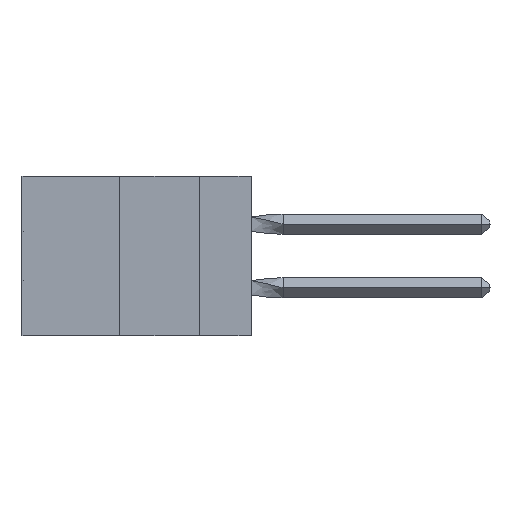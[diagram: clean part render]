
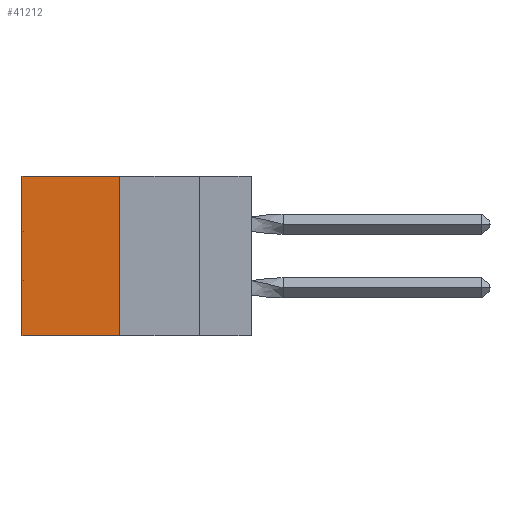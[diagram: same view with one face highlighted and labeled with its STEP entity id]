
A CAD part, left-side view. The second image highlights one B-rep face of the part: STEP entity #41212.
In plain terms, the highlighted planar face has unit normal (-1, 0, 0).
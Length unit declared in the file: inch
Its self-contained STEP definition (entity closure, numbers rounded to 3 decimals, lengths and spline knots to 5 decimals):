
#1384 = VERTEX_POINT ( 'NONE', #13139 ) ;
#1548 = LINE ( 'NONE', #21784, #15358 ) ;
#1562 = EDGE_CURVE ( 'NONE', #7573, #21816, #4903, .T. ) ;
#2944 = DIRECTION ( 'NONE',  ( 0., 0., -1. ) ) ;
#3630 = LINE ( 'NONE', #15816, #15417 ) ;
#4903 = LINE ( 'NONE', #5093, #20805 ) ;
#4969 = EDGE_LOOP ( 'NONE', ( #41977, #9953, #30046, #12550 ) ) ;
#5093 = CARTESIAN_POINT ( 'NONE',  ( 0.305, 0.413, -0.5 ) ) ;
#7357 = DIRECTION ( 'NONE',  ( 0., 0., -1. ) ) ;
#7573 = VERTEX_POINT ( 'NONE', #14237 ) ;
#8630 = DIRECTION ( 'NONE',  ( 0., 0., -1. ) ) ;
#9953 = ORIENTED_EDGE ( 'NONE', *, *, #1562, .F. ) ;
#12550 = ORIENTED_EDGE ( 'NONE', *, *, #19380, .T. ) ;
#12794 = DIRECTION ( 'NONE',  ( 1., 0., 0. ) ) ;
#13139 = CARTESIAN_POINT ( 'NONE',  ( 0.305, 0.72, 0. ) ) ;
#14204 = CARTESIAN_POINT ( 'NONE',  ( 0.305, 0.72, -0.5 ) ) ;
#14237 = CARTESIAN_POINT ( 'NONE',  ( 0.305, 0.413, -0.5 ) ) ;
#14244 = AXIS2_PLACEMENT_3D ( 'NONE', #20266, #12794, #7357 ) ;
#15358 = VECTOR ( 'NONE', #8630, 39.37008 ) ;
#15417 = VECTOR ( 'NONE', #2944, 39.37008 ) ;
#15816 = CARTESIAN_POINT ( 'NONE',  ( 0.305, 0.72, -0.5 ) ) ;
#19380 = EDGE_CURVE ( 'NONE', #39048, #1384, #26213, .T. ) ;
#20266 = CARTESIAN_POINT ( 'NONE',  ( 0.305, 0.413, -0.5 ) ) ;
#20805 = VECTOR ( 'NONE', #31602, 39.37008 ) ;
#21784 = CARTESIAN_POINT ( 'NONE',  ( 0.305, 0.413, -0.5 ) ) ;
#21816 = VERTEX_POINT ( 'NONE', #14204 ) ;
#22784 = PLANE ( 'NONE',  #14244 ) ;
#25388 = FACE_OUTER_BOUND ( 'NONE', #4969, .T. ) ;
#26213 = LINE ( 'NONE', #32638, #33430 ) ;
#26299 = EDGE_CURVE ( 'NONE', #1384, #21816, #3630, .T. ) ;
#28317 = CARTESIAN_POINT ( 'NONE',  ( 0.305, 0.413, 0. ) ) ;
#30046 = ORIENTED_EDGE ( 'NONE', *, *, #32184, .F. ) ;
#31602 = DIRECTION ( 'NONE',  ( 0., 1., 0. ) ) ;
#32184 = EDGE_CURVE ( 'NONE', #39048, #7573, #1548, .T. ) ;
#32215 = DIRECTION ( 'NONE',  ( 0., 1., 0. ) ) ;
#32638 = CARTESIAN_POINT ( 'NONE',  ( 0.305, 0.413, 0. ) ) ;
#33430 = VECTOR ( 'NONE', #32215, 39.37008 ) ;
#39048 = VERTEX_POINT ( 'NONE', #28317 ) ;
#41212 = ADVANCED_FACE ( 'NONE', ( #25388 ), #22784, .F. ) ;
#41977 = ORIENTED_EDGE ( 'NONE', *, *, #26299, .T. ) ;
